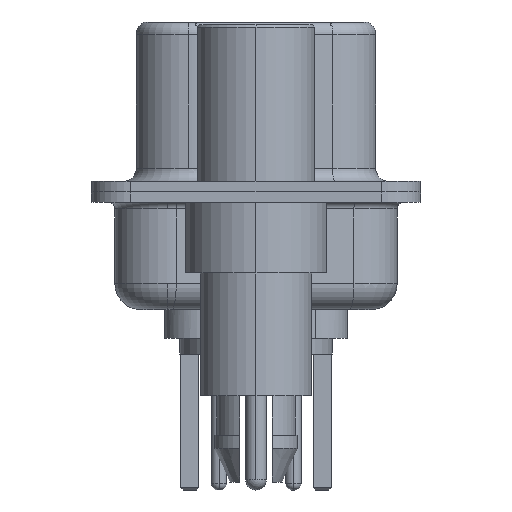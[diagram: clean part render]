
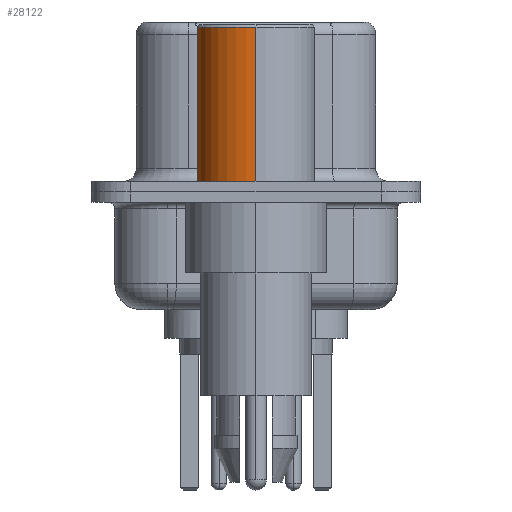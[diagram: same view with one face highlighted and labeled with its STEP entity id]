
A CAD part, left-side view. The second image highlights one B-rep face of the part: STEP entity #28122.
In plain terms, the highlighted cylindrical face has radius 2.25 mm (diameter 4.5 mm), a partial arc.
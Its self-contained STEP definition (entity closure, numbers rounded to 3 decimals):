
#1272 = CARTESIAN_POINT ( 'NONE',  ( 2.25, 0., 6.3 ) ) ;
#2063 = CARTESIAN_POINT ( 'NONE',  ( 2.25, 0., 0.581 ) ) ;
#2608 = VERTEX_POINT ( 'NONE', #23516 ) ;
#2812 = DIRECTION ( 'NONE',  ( 0., 0., 1. ) ) ;
#3127 = CIRCLE ( 'NONE', #26939, 2.25 ) ;
#3505 = EDGE_CURVE ( 'NONE', #13515, #17773, #19988, .T. ) ;
#4196 = CIRCLE ( 'NONE', #10052, 2.25 ) ;
#4677 = CARTESIAN_POINT ( 'NONE',  ( -2.25, 0., 6.3 ) ) ;
#5537 = AXIS2_PLACEMENT_3D ( 'NONE', #14568, #7773, #27731 ) ;
#5897 = CARTESIAN_POINT ( 'NONE',  ( 2.25, 0., 0.4 ) ) ;
#6331 = CARTESIAN_POINT ( 'NONE',  ( 0., 0., 6.3 ) ) ;
#6452 = ORIENTED_EDGE ( 'NONE', *, *, #23449, .T. ) ;
#7773 = DIRECTION ( 'NONE',  ( 0., 0., 1. ) ) ;
#7903 = ORIENTED_EDGE ( 'NONE', *, *, #16706, .F. ) ;
#8607 = CARTESIAN_POINT ( 'NONE',  ( 0., 0., 0.4 ) ) ;
#8638 = DIRECTION ( 'NONE',  ( 1., 0., 0. ) ) ;
#10052 = AXIS2_PLACEMENT_3D ( 'NONE', #8607, #24032, #10857 ) ;
#10411 = LINE ( 'NONE', #21254, #25900 ) ;
#10857 = DIRECTION ( 'NONE',  ( 1., 0., 0. ) ) ;
#11283 = EDGE_LOOP ( 'NONE', ( #17495, #6452, #7903, #18974 ) ) ;
#13484 = VECTOR ( 'NONE', #2812, 1000. ) ;
#13515 = VERTEX_POINT ( 'NONE', #5897 ) ;
#14568 = CARTESIAN_POINT ( 'NONE',  ( 0., 0., 0.581 ) ) ;
#16706 = EDGE_CURVE ( 'NONE', #17773, #25768, #3127, .T. ) ;
#17495 = ORIENTED_EDGE ( 'NONE', *, *, #19068, .T. ) ;
#17773 = VERTEX_POINT ( 'NONE', #1272 ) ;
#17969 = FACE_OUTER_BOUND ( 'NONE', #11283, .T. ) ;
#18974 = ORIENTED_EDGE ( 'NONE', *, *, #3505, .F. ) ;
#18975 = DIRECTION ( 'NONE',  ( 0., 0., 1. ) ) ;
#19068 = EDGE_CURVE ( 'NONE', #13515, #2608, #4196, .T. ) ;
#19988 = LINE ( 'NONE', #2063, #13484 ) ;
#21254 = CARTESIAN_POINT ( 'NONE',  ( -2.25, 0., 0.581 ) ) ;
#21848 = DIRECTION ( 'NONE',  ( 0., 0., 1. ) ) ;
#23449 = EDGE_CURVE ( 'NONE', #2608, #25768, #10411, .T. ) ;
#23516 = CARTESIAN_POINT ( 'NONE',  ( -2.25, 0., 0.4 ) ) ;
#24032 = DIRECTION ( 'NONE',  ( 0., 0., 1. ) ) ;
#25768 = VERTEX_POINT ( 'NONE', #4677 ) ;
#25900 = VECTOR ( 'NONE', #18975, 1000. ) ;
#26939 = AXIS2_PLACEMENT_3D ( 'NONE', #6331, #21848, #8638 ) ;
#27731 = DIRECTION ( 'NONE',  ( 1., 0., 0. ) ) ;
#28122 = ADVANCED_FACE ( 'NONE', ( #17969 ), #28231, .T. ) ;
#28231 = CYLINDRICAL_SURFACE ( 'NONE', #5537, 2.25 ) ;
